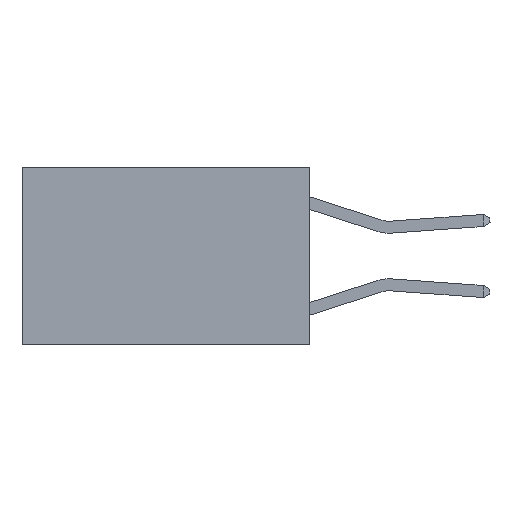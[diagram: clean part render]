
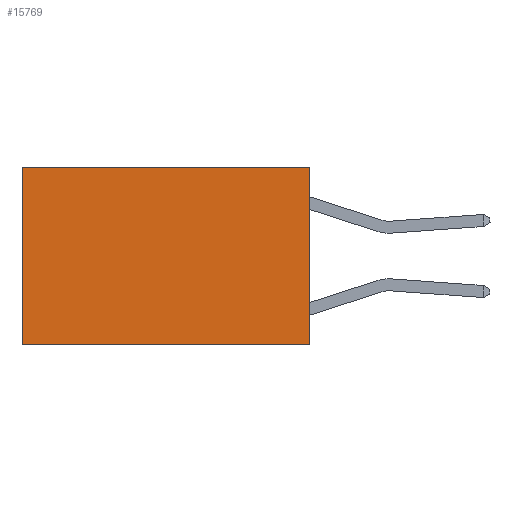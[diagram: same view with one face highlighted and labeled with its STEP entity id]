
A CAD part, left-side view. The second image highlights one B-rep face of the part: STEP entity #15769.
In plain terms, the highlighted planar face has unit normal (-1, 0, 0).
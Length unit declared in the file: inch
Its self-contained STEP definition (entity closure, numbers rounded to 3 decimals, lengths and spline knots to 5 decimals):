
#1942 = VERTEX_POINT ( 'NONE', #8540 ) ;
#2057 = CARTESIAN_POINT ( 'NONE',  ( 0.2625, 0., 0. ) ) ;
#2396 = VERTEX_POINT ( 'NONE', #22231 ) ;
#2756 = EDGE_CURVE ( 'NONE', #26376, #21784, #13409, .T. ) ;
#6374 = DIRECTION ( 'NONE',  ( 0., 0., -1. ) ) ;
#6759 = EDGE_CURVE ( 'NONE', #2396, #1942, #17577, .T. ) ;
#7032 = ORIENTED_EDGE ( 'NONE', *, *, #2756, .T. ) ;
#7044 = CARTESIAN_POINT ( 'NONE',  ( 0.2625, 0., -0.37 ) ) ;
#7821 = CARTESIAN_POINT ( 'NONE',  ( 0.2625, 0., 0. ) ) ;
#8427 = DIRECTION ( 'NONE',  ( 0., 0., -1. ) ) ;
#8540 = CARTESIAN_POINT ( 'NONE',  ( 0.2625, 0., -0.37 ) ) ;
#8897 = ORIENTED_EDGE ( 'NONE', *, *, #9395, .T. ) ;
#9395 = EDGE_CURVE ( 'NONE', #2396, #26376, #23853, .T. ) ;
#10614 = AXIS2_PLACEMENT_3D ( 'NONE', #2057, #13978, #18672 ) ;
#11437 = LINE ( 'NONE', #7044, #14730 ) ;
#11818 = VECTOR ( 'NONE', #6374, 39.37008 ) ;
#13409 = LINE ( 'NONE', #22487, #28921 ) ;
#13978 = DIRECTION ( 'NONE',  ( 1., 0., 0. ) ) ;
#14127 = PLANE ( 'NONE',  #10614 ) ;
#14504 = EDGE_LOOP ( 'NONE', ( #7032, #28738, #29024, #8897 ) ) ;
#14566 = VECTOR ( 'NONE', #16898, 39.37008 ) ;
#14730 = VECTOR ( 'NONE', #25342, 39.37008 ) ;
#15769 = ADVANCED_FACE ( 'NONE', ( #20487 ), #14127, .F. ) ;
#16611 = CARTESIAN_POINT ( 'NONE',  ( 0.2625, 0.6, 0. ) ) ;
#16898 = DIRECTION ( 'NONE',  ( 0., 1., 0. ) ) ;
#17577 = LINE ( 'NONE', #24239, #11818 ) ;
#18672 = DIRECTION ( 'NONE',  ( 0., 0., -1. ) ) ;
#20487 = FACE_OUTER_BOUND ( 'NONE', #14504, .T. ) ;
#20505 = CARTESIAN_POINT ( 'NONE',  ( 0.2625, 0.6, -0.37 ) ) ;
#21763 = EDGE_CURVE ( 'NONE', #1942, #21784, #11437, .T. ) ;
#21784 = VERTEX_POINT ( 'NONE', #20505 ) ;
#22231 = CARTESIAN_POINT ( 'NONE',  ( 0.2625, 0., 0. ) ) ;
#22487 = CARTESIAN_POINT ( 'NONE',  ( 0.2625, 0.6, 0. ) ) ;
#23853 = LINE ( 'NONE', #7821, #14566 ) ;
#24239 = CARTESIAN_POINT ( 'NONE',  ( 0.2625, 0., 0. ) ) ;
#25342 = DIRECTION ( 'NONE',  ( 0., 1., 0. ) ) ;
#26376 = VERTEX_POINT ( 'NONE', #16611 ) ;
#28738 = ORIENTED_EDGE ( 'NONE', *, *, #21763, .F. ) ;
#28921 = VECTOR ( 'NONE', #8427, 39.37008 ) ;
#29024 = ORIENTED_EDGE ( 'NONE', *, *, #6759, .F. ) ;
